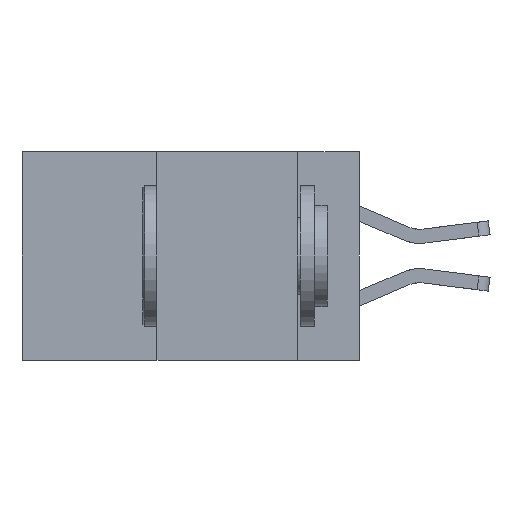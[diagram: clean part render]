
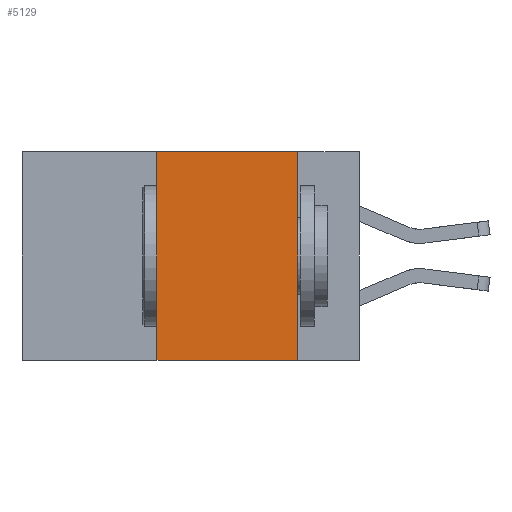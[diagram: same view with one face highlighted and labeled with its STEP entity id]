
A CAD part, left-side view. The second image highlights one B-rep face of the part: STEP entity #5129.
In plain terms, the highlighted planar face has unit normal (-1, 0, 0).
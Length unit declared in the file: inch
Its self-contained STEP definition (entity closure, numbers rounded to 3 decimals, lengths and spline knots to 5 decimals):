
#1 = DIRECTION ( 'NONE',  ( 0., -1., 0. ) ) ;
#312 = ORIENTED_EDGE ( 'NONE', *, *, #6153, .T. ) ;
#883 = LINE ( 'NONE', #8752, #2716 ) ;
#966 = DIRECTION ( 'NONE',  ( 0., 0., 1. ) ) ;
#2341 = DIRECTION ( 'NONE',  ( 0., 0., -1. ) ) ;
#2479 = EDGE_CURVE ( 'NONE', #4602, #4387, #9085, .T. ) ;
#2543 = DIRECTION ( 'NONE',  ( 0., 0., -1. ) ) ;
#2716 = VECTOR ( 'NONE', #1, 39.37008 ) ;
#2827 = CARTESIAN_POINT ( 'NONE',  ( 0., 0.36, 0. ) ) ;
#3197 = VERTEX_POINT ( 'NONE', #9174 ) ;
#3419 = ORIENTED_EDGE ( 'NONE', *, *, #3899, .F. ) ;
#3685 = VECTOR ( 'NONE', #5567, 39.37008 ) ;
#3899 = EDGE_CURVE ( 'NONE', #3197, #4602, #4624, .T. ) ;
#4308 = VECTOR ( 'NONE', #966, 39.37008 ) ;
#4387 = VERTEX_POINT ( 'NONE', #5696 ) ;
#4602 = VERTEX_POINT ( 'NONE', #2827 ) ;
#4624 = LINE ( 'NONE', #6222, #4308 ) ;
#4860 = VERTEX_POINT ( 'NONE', #7396 ) ;
#5070 = EDGE_LOOP ( 'NONE', ( #11051, #8256, #3419, #312 ) ) ;
#5129 = ADVANCED_FACE ( 'NONE', ( #6473 ), #5775, .F. ) ;
#5567 = DIRECTION ( 'NONE',  ( 0., -1., 0. ) ) ;
#5696 = CARTESIAN_POINT ( 'NONE',  ( 0., 0.11, 0. ) ) ;
#5775 = PLANE ( 'NONE',  #13934 ) ;
#5815 = CARTESIAN_POINT ( 'NONE',  ( 0., 0.6, 0. ) ) ;
#6153 = EDGE_CURVE ( 'NONE', #3197, #4860, #883, .T. ) ;
#6222 = CARTESIAN_POINT ( 'NONE',  ( 0., 0.36, 0. ) ) ;
#6473 = FACE_OUTER_BOUND ( 'NONE', #5070, .T. ) ;
#7020 = LINE ( 'NONE', #8807, #11064 ) ;
#7396 = CARTESIAN_POINT ( 'NONE',  ( 0., 0.11, -0.37 ) ) ;
#7569 = EDGE_CURVE ( 'NONE', #4387, #4860, #7020, .T. ) ;
#8256 = ORIENTED_EDGE ( 'NONE', *, *, #2479, .F. ) ;
#8752 = CARTESIAN_POINT ( 'NONE',  ( 0., 0.6, -0.37 ) ) ;
#8807 = CARTESIAN_POINT ( 'NONE',  ( 0., 0.11, 0. ) ) ;
#9085 = LINE ( 'NONE', #11955, #3685 ) ;
#9131 = DIRECTION ( 'NONE',  ( 1., 0., 0. ) ) ;
#9174 = CARTESIAN_POINT ( 'NONE',  ( 0., 0.36, -0.37 ) ) ;
#11051 = ORIENTED_EDGE ( 'NONE', *, *, #7569, .F. ) ;
#11064 = VECTOR ( 'NONE', #2341, 39.37008 ) ;
#11955 = CARTESIAN_POINT ( 'NONE',  ( 0., 0.6, 0. ) ) ;
#13934 = AXIS2_PLACEMENT_3D ( 'NONE', #5815, #9131, #2543 ) ;
